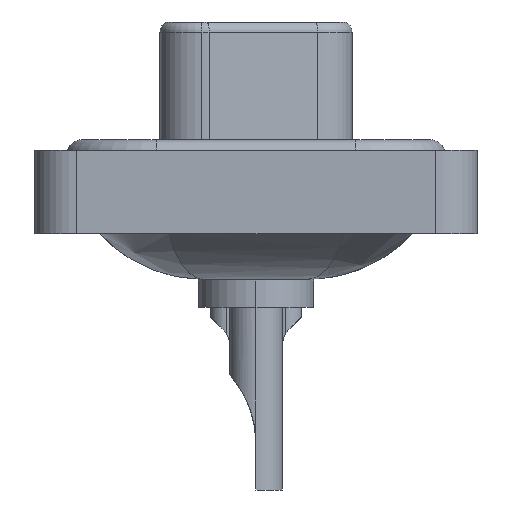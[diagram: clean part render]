
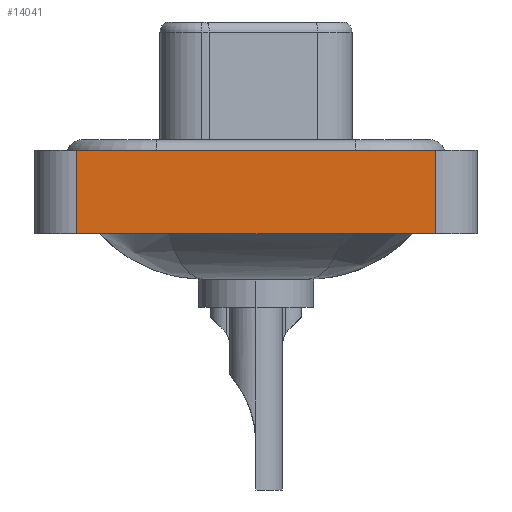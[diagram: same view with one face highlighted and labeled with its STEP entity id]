
A CAD part, left-side view. The second image highlights one B-rep face of the part: STEP entity #14041.
In plain terms, the highlighted planar face has unit normal (-1, 0, 0).
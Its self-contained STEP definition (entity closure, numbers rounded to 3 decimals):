
#477 = VECTOR ( 'NONE', #11111, 1000. ) ;
#916 = FACE_OUTER_BOUND ( 'NONE', #939, .T. ) ;
#939 = EDGE_LOOP ( 'NONE', ( #5444, #2691, #19428, #3310 ) ) ;
#1213 = VERTEX_POINT ( 'NONE', #3517 ) ;
#1292 = PLANE ( 'NONE',  #8567 ) ;
#1688 = LINE ( 'NONE', #15500, #7103 ) ;
#2399 = CARTESIAN_POINT ( 'NONE',  ( -7.3, -8.55, -3.6 ) ) ;
#2417 = EDGE_CURVE ( 'NONE', #6918, #9884, #17202, .T. ) ;
#2490 = DIRECTION ( 'NONE',  ( 0., 0., 1. ) ) ;
#2691 = ORIENTED_EDGE ( 'NONE', *, *, #12645, .F. ) ;
#2860 = EDGE_CURVE ( 'NONE', #6918, #12293, #1688, .T. ) ;
#3310 = ORIENTED_EDGE ( 'NONE', *, *, #2860, .T. ) ;
#3517 = CARTESIAN_POINT ( 'NONE',  ( -7.3, -8.55, 0.4 ) ) ;
#3882 = EDGE_CURVE ( 'NONE', #12293, #1213, #18638, .T. ) ;
#4161 = DIRECTION ( 'NONE',  ( -1., 0., 0. ) ) ;
#4542 = VECTOR ( 'NONE', #12037, 1000. ) ;
#5006 = CARTESIAN_POINT ( 'NONE',  ( -7.3, 8.55, 0.4 ) ) ;
#5090 = CARTESIAN_POINT ( 'NONE',  ( -7.3, -8.55, -3.6 ) ) ;
#5444 = ORIENTED_EDGE ( 'NONE', *, *, #3882, .T. ) ;
#6024 = LINE ( 'NONE', #9366, #4542 ) ;
#6918 = VERTEX_POINT ( 'NONE', #8295 ) ;
#7103 = VECTOR ( 'NONE', #15402, 1000. ) ;
#7412 = VECTOR ( 'NONE', #15424, 1000. ) ;
#8020 = CARTESIAN_POINT ( 'NONE',  ( -7.3, -8.55, -3.6 ) ) ;
#8295 = CARTESIAN_POINT ( 'NONE',  ( -7.3, 8.55, -3.6 ) ) ;
#8567 = AXIS2_PLACEMENT_3D ( 'NONE', #2399, #4161, #2490 ) ;
#9366 = CARTESIAN_POINT ( 'NONE',  ( -7.3, -8.55, 0.4 ) ) ;
#9884 = VERTEX_POINT ( 'NONE', #5006 ) ;
#11111 = DIRECTION ( 'NONE',  ( 0., 0., 1. ) ) ;
#12037 = DIRECTION ( 'NONE',  ( 0., -1., 0. ) ) ;
#12293 = VERTEX_POINT ( 'NONE', #8020 ) ;
#12645 = EDGE_CURVE ( 'NONE', #9884, #1213, #6024, .T. ) ;
#14041 = ADVANCED_FACE ( 'NONE', ( #916 ), #1292, .T. ) ;
#15402 = DIRECTION ( 'NONE',  ( 0., -1., 0. ) ) ;
#15424 = DIRECTION ( 'NONE',  ( 0., 0., 1. ) ) ;
#15500 = CARTESIAN_POINT ( 'NONE',  ( -7.3, -8.55, -3.6 ) ) ;
#17202 = LINE ( 'NONE', #18610, #7412 ) ;
#18610 = CARTESIAN_POINT ( 'NONE',  ( -7.3, 8.55, -3.6 ) ) ;
#18638 = LINE ( 'NONE', #5090, #477 ) ;
#19428 = ORIENTED_EDGE ( 'NONE', *, *, #2417, .F. ) ;
